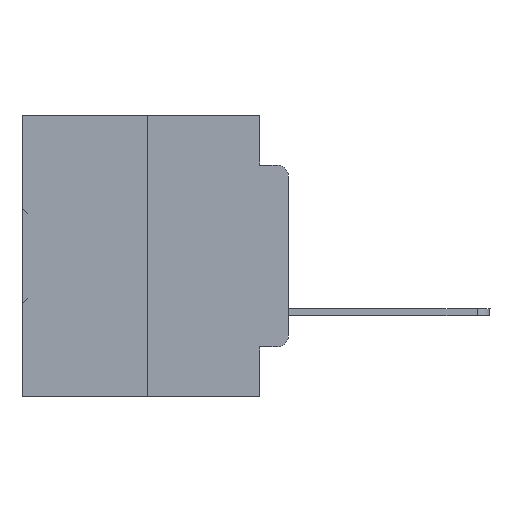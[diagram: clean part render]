
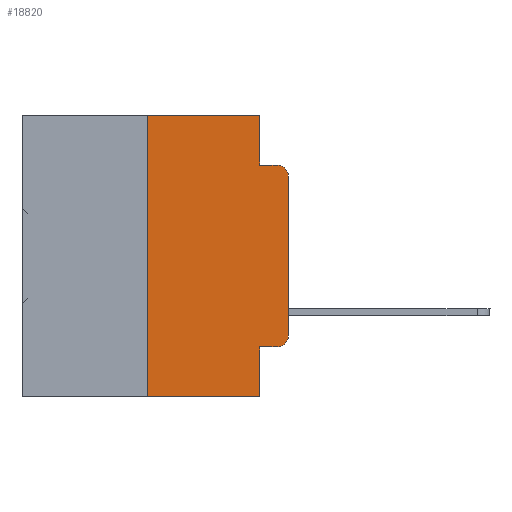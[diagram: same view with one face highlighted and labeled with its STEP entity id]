
A CAD part, left-side view. The second image highlights one B-rep face of the part: STEP entity #18820.
In plain terms, the highlighted planar face has unit normal (-1, 0, 0).
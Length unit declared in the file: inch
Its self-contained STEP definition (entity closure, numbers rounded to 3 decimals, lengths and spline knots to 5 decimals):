
#570 = DIRECTION ( 'NONE',  ( -1., 0., 0. ) ) ;
#609 = ORIENTED_EDGE ( 'NONE', *, *, #7251, .T. ) ;
#956 = VECTOR ( 'NONE', #24378, 39.37008 ) ;
#1186 = ORIENTED_EDGE ( 'NONE', *, *, #14003, .F. ) ;
#1821 = DIRECTION ( 'NONE',  ( 0., 0., 1. ) ) ;
#3914 = VERTEX_POINT ( 'NONE', #18270 ) ;
#4133 = CARTESIAN_POINT ( 'NONE',  ( 0., 0.051, 0. ) ) ;
#4184 = EDGE_CURVE ( 'NONE', #4694, #37334, #25330, .T. ) ;
#4206 = EDGE_CURVE ( 'NONE', #21847, #3914, #33999, .T. ) ;
#4694 = VERTEX_POINT ( 'NONE', #33648 ) ;
#4760 = DIRECTION ( 'NONE',  ( -1., 0., 0. ) ) ;
#5799 = LINE ( 'NONE', #37665, #23708 ) ;
#7180 = DIRECTION ( 'NONE',  ( 0., 0., -1. ) ) ;
#7251 = EDGE_CURVE ( 'NONE', #36066, #35959, #10290, .T. ) ;
#7501 = LINE ( 'NONE', #15675, #18118 ) ;
#8048 = CARTESIAN_POINT ( 'NONE',  ( 0., 0.051, -0.4115 ) ) ;
#8111 = ORIENTED_EDGE ( 'NONE', *, *, #4184, .T. ) ;
#8703 = LINE ( 'NONE', #26946, #956 ) ;
#9287 = ORIENTED_EDGE ( 'NONE', *, *, #4206, .F. ) ;
#9389 = CARTESIAN_POINT ( 'NONE',  ( 0., 0.473, 0. ) ) ;
#9546 = FACE_OUTER_BOUND ( 'NONE', #36458, .T. ) ;
#10205 = VERTEX_POINT ( 'NONE', #20398 ) ;
#10290 = LINE ( 'NONE', #28773, #20401 ) ;
#10651 = CARTESIAN_POINT ( 'NONE',  ( 0., 0.25, 0. ) ) ;
#10669 = VECTOR ( 'NONE', #27461, 39.37008 ) ;
#11130 = VERTEX_POINT ( 'NONE', #36172 ) ;
#11568 = VERTEX_POINT ( 'NONE', #37545 ) ;
#12080 = CARTESIAN_POINT ( 'NONE',  ( 0., 0.02, -0.3915 ) ) ;
#12329 = DIRECTION ( 'NONE',  ( 0., -1., 0. ) ) ;
#12563 = EDGE_CURVE ( 'NONE', #10205, #4694, #30665, .T. ) ;
#13669 = EDGE_CURVE ( 'NONE', #11568, #37334, #5799, .T. ) ;
#13849 = ORIENTED_EDGE ( 'NONE', *, *, #32933, .T. ) ;
#14003 = EDGE_CURVE ( 'NONE', #3914, #11130, #34636, .T. ) ;
#14608 = DIRECTION ( 'NONE',  ( 0., 0., 1. ) ) ;
#15406 = CARTESIAN_POINT ( 'NONE',  ( 0., 0.25, -0.5 ) ) ;
#15416 = DIRECTION ( 'NONE',  ( 1., 0., 0. ) ) ;
#15537 = VECTOR ( 'NONE', #14608, 39.37008 ) ;
#15675 = CARTESIAN_POINT ( 'NONE',  ( 0., 0.473, -0.5 ) ) ;
#15900 = AXIS2_PLACEMENT_3D ( 'NONE', #28107, #4760, #7180 ) ;
#16451 = CARTESIAN_POINT ( 'NONE',  ( 0., 0.02, -0.4115 ) ) ;
#16650 = ORIENTED_EDGE ( 'NONE', *, *, #27174, .F. ) ;
#18118 = VECTOR ( 'NONE', #18854, 39.37008 ) ;
#18240 = CARTESIAN_POINT ( 'NONE',  ( 0., 0.051, -0.5 ) ) ;
#18270 = CARTESIAN_POINT ( 'NONE',  ( 0., 0.25, 0. ) ) ;
#18820 = ADVANCED_FACE ( 'NONE', ( #9546 ), #27573, .F. ) ;
#18854 = DIRECTION ( 'NONE',  ( 0., -1., 0. ) ) ;
#19927 = CARTESIAN_POINT ( 'NONE',  ( 0., 0.02, -0.0885 ) ) ;
#20044 = DIRECTION ( 'NONE',  ( 0., -1., 0. ) ) ;
#20398 = CARTESIAN_POINT ( 'NONE',  ( 0., 0., -0.3915 ) ) ;
#20401 = VECTOR ( 'NONE', #20044, 39.37008 ) ;
#21058 = DIRECTION ( 'NONE',  ( 0., 0., -1. ) ) ;
#21539 = EDGE_CURVE ( 'NONE', #11130, #11568, #32214, .T. ) ;
#21847 = VERTEX_POINT ( 'NONE', #15406 ) ;
#22290 = VECTOR ( 'NONE', #12329, 39.37008 ) ;
#23500 = ORIENTED_EDGE ( 'NONE', *, *, #31968, .T. ) ;
#23708 = VECTOR ( 'NONE', #37404, 39.37008 ) ;
#24378 = DIRECTION ( 'NONE',  ( 0., 0., -1. ) ) ;
#25330 = CIRCLE ( 'NONE', #15900, 0.02 ) ;
#25515 = ORIENTED_EDGE ( 'NONE', *, *, #12563, .T. ) ;
#26946 = CARTESIAN_POINT ( 'NONE',  ( 0., 0.051, 0. ) ) ;
#27174 = EDGE_CURVE ( 'NONE', #36066, #32869, #8703, .T. ) ;
#27461 = DIRECTION ( 'NONE',  ( 0., 0., -1. ) ) ;
#27573 = PLANE ( 'NONE',  #33466 ) ;
#28107 = CARTESIAN_POINT ( 'NONE',  ( 0., 0.02, -0.1085 ) ) ;
#28773 = CARTESIAN_POINT ( 'NONE',  ( 0., 0.051, -0.4115 ) ) ;
#29160 = ORIENTED_EDGE ( 'NONE', *, *, #13669, .F. ) ;
#29240 = ORIENTED_EDGE ( 'NONE', *, *, #21539, .F. ) ;
#29957 = VECTOR ( 'NONE', #1821, 39.37008 ) ;
#30500 = CARTESIAN_POINT ( 'NONE',  ( 0., 0.473, 0. ) ) ;
#30665 = LINE ( 'NONE', #32125, #15537 ) ;
#31968 = EDGE_CURVE ( 'NONE', #21847, #32869, #7501, .T. ) ;
#32125 = CARTESIAN_POINT ( 'NONE',  ( 0., 0., 0. ) ) ;
#32198 = CIRCLE ( 'NONE', #37125, 0.02 ) ;
#32214 = LINE ( 'NONE', #4133, #10669 ) ;
#32869 = VERTEX_POINT ( 'NONE', #18240 ) ;
#32933 = EDGE_CURVE ( 'NONE', #35959, #10205, #32198, .T. ) ;
#33466 = AXIS2_PLACEMENT_3D ( 'NONE', #30500, #15416, #36235 ) ;
#33648 = CARTESIAN_POINT ( 'NONE',  ( 0., 0., -0.1085 ) ) ;
#33999 = LINE ( 'NONE', #10651, #29957 ) ;
#34636 = LINE ( 'NONE', #9389, #22290 ) ;
#35959 = VERTEX_POINT ( 'NONE', #16451 ) ;
#36066 = VERTEX_POINT ( 'NONE', #8048 ) ;
#36172 = CARTESIAN_POINT ( 'NONE',  ( 0., 0.051, 0. ) ) ;
#36235 = DIRECTION ( 'NONE',  ( 0., 0., -1. ) ) ;
#36458 = EDGE_LOOP ( 'NONE', ( #25515, #8111, #29160, #29240, #1186, #9287, #23500, #16650, #609, #13849 ) ) ;
#37125 = AXIS2_PLACEMENT_3D ( 'NONE', #12080, #570, #21058 ) ;
#37334 = VERTEX_POINT ( 'NONE', #19927 ) ;
#37404 = DIRECTION ( 'NONE',  ( 0., -1., 0. ) ) ;
#37545 = CARTESIAN_POINT ( 'NONE',  ( 0., 0.051, -0.0885 ) ) ;
#37665 = CARTESIAN_POINT ( 'NONE',  ( 0., 0.051, -0.0885 ) ) ;
